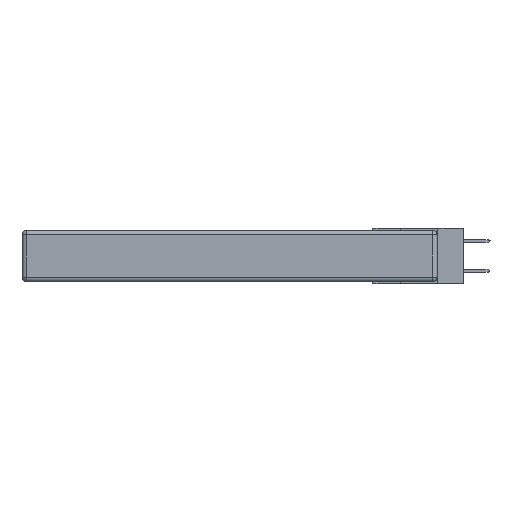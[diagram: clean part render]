
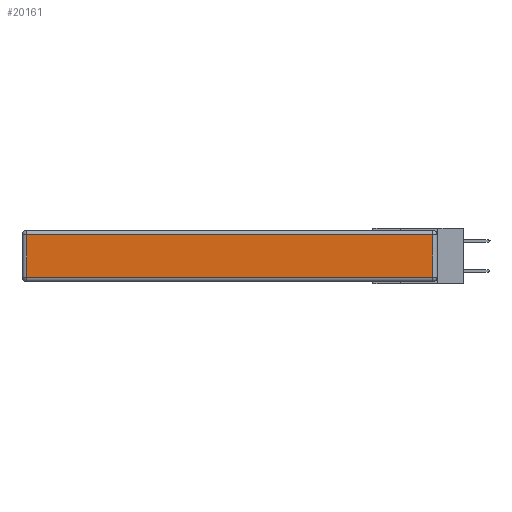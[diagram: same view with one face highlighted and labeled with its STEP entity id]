
A CAD part, left-side view. The second image highlights one B-rep face of the part: STEP entity #20161.
In plain terms, the highlighted planar face has unit normal (-1, 0, 0).
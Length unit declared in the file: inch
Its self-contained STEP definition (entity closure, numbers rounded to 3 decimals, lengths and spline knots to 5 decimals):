
#2313 = CARTESIAN_POINT ( 'NONE',  ( 0., 2.72, -0.313 ) ) ;
#2699 = DIRECTION ( 'NONE',  ( 0., 0., 1. ) ) ;
#3222 = LINE ( 'NONE', #22159, #8126 ) ;
#3593 = ORIENTED_EDGE ( 'NONE', *, *, #23648, .T. ) ;
#4925 = VERTEX_POINT ( 'NONE', #11512 ) ;
#5159 = LINE ( 'NONE', #25884, #15597 ) ;
#6359 = CARTESIAN_POINT ( 'NONE',  ( 0., 0., -0.343 ) ) ;
#7622 = CARTESIAN_POINT ( 'NONE',  ( 0., 0.03, -0.313 ) ) ;
#7661 = EDGE_LOOP ( 'NONE', ( #16952, #3593, #22026, #12961 ) ) ;
#7812 = FACE_OUTER_BOUND ( 'NONE', #7661, .T. ) ;
#8008 = CARTESIAN_POINT ( 'NONE',  ( 0., 0.03, -0.03 ) ) ;
#8126 = VECTOR ( 'NONE', #12346, 39.37008 ) ;
#8381 = PLANE ( 'NONE',  #14712 ) ;
#10433 = DIRECTION ( 'NONE',  ( 0., 0., -1. ) ) ;
#11512 = CARTESIAN_POINT ( 'NONE',  ( 0., 2.72, -0.03 ) ) ;
#12346 = DIRECTION ( 'NONE',  ( 0., -1., 0. ) ) ;
#12619 = DIRECTION ( 'NONE',  ( -1., 0., 0. ) ) ;
#12961 = ORIENTED_EDGE ( 'NONE', *, *, #20786, .T. ) ;
#14059 = VERTEX_POINT ( 'NONE', #2313 ) ;
#14105 = VERTEX_POINT ( 'NONE', #7622 ) ;
#14712 = AXIS2_PLACEMENT_3D ( 'NONE', #6359, #12619, #20947 ) ;
#15122 = VECTOR ( 'NONE', #10433, 39.37008 ) ;
#15597 = VECTOR ( 'NONE', #2699, 39.37008 ) ;
#16151 = VECTOR ( 'NONE', #24542, 39.37008 ) ;
#16403 = CARTESIAN_POINT ( 'NONE',  ( 0., 2.75, -0.03 ) ) ;
#16952 = ORIENTED_EDGE ( 'NONE', *, *, #19890, .T. ) ;
#16966 = EDGE_CURVE ( 'NONE', #19206, #4925, #21773, .T. ) ;
#19206 = VERTEX_POINT ( 'NONE', #8008 ) ;
#19890 = EDGE_CURVE ( 'NONE', #14059, #14105, #3222, .T. ) ;
#20161 = ADVANCED_FACE ( 'NONE', ( #7812 ), #8381, .T. ) ;
#20786 = EDGE_CURVE ( 'NONE', #4925, #14059, #26649, .T. ) ;
#20947 = DIRECTION ( 'NONE',  ( 0., 0., 1. ) ) ;
#21773 = LINE ( 'NONE', #16403, #16151 ) ;
#22026 = ORIENTED_EDGE ( 'NONE', *, *, #16966, .T. ) ;
#22159 = CARTESIAN_POINT ( 'NONE',  ( 0., 0., -0.313 ) ) ;
#23648 = EDGE_CURVE ( 'NONE', #14105, #19206, #5159, .T. ) ;
#24542 = DIRECTION ( 'NONE',  ( 0., 1., 0. ) ) ;
#25223 = CARTESIAN_POINT ( 'NONE',  ( 0., 2.72, -0.343 ) ) ;
#25884 = CARTESIAN_POINT ( 'NONE',  ( 0., 0.03, -0.343 ) ) ;
#26649 = LINE ( 'NONE', #25223, #15122 ) ;
